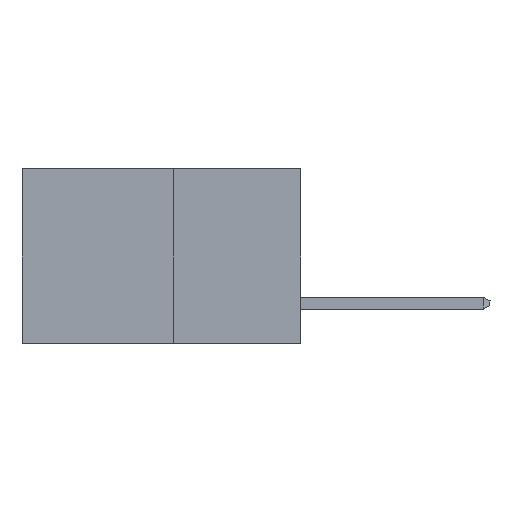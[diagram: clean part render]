
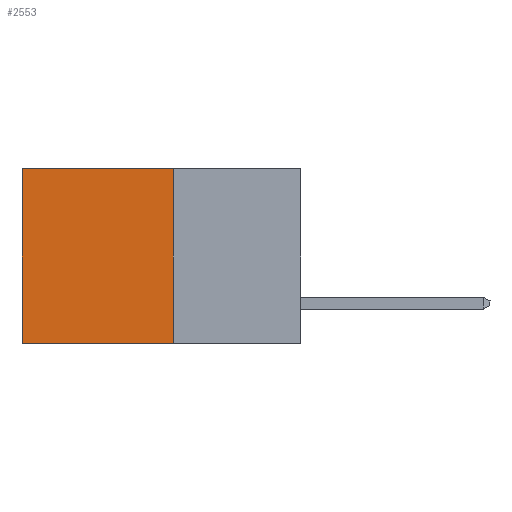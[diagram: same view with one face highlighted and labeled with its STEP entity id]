
A CAD part, left-side view. The second image highlights one B-rep face of the part: STEP entity #2553.
In plain terms, the highlighted planar face has unit normal (-1, 0, 0).
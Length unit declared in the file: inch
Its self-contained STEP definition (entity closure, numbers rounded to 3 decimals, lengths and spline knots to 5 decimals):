
#209 = LINE ( 'NONE', #13636, #10905 ) ;
#876 = EDGE_CURVE ( 'NONE', #1116, #26297, #20223, .T. ) ;
#1116 = VERTEX_POINT ( 'NONE', #6637 ) ;
#1895 = VECTOR ( 'NONE', #26187, 39.37008 ) ;
#2246 = VECTOR ( 'NONE', #16918, 39.37008 ) ;
#2553 = ADVANCED_FACE ( 'NONE', ( #9293 ), #8176, .F. ) ;
#4101 = ORIENTED_EDGE ( 'NONE', *, *, #876, .F. ) ;
#5620 = CARTESIAN_POINT ( 'NONE',  ( 0.277, 0.27, -0.37 ) ) ;
#5888 = DIRECTION ( 'NONE',  ( 0., 0., -1. ) ) ;
#6032 = CARTESIAN_POINT ( 'NONE',  ( 0.277, 0.27, 0. ) ) ;
#6637 = CARTESIAN_POINT ( 'NONE',  ( 0.277, 0.27, 0. ) ) ;
#7796 = ORIENTED_EDGE ( 'NONE', *, *, #14013, .F. ) ;
#7887 = EDGE_CURVE ( 'NONE', #14199, #18942, #19100, .T. ) ;
#8090 = EDGE_LOOP ( 'NONE', ( #9968, #7796, #4101, #16827 ) ) ;
#8176 = PLANE ( 'NONE',  #21762 ) ;
#9293 = FACE_OUTER_BOUND ( 'NONE', #8090, .T. ) ;
#9968 = ORIENTED_EDGE ( 'NONE', *, *, #7887, .T. ) ;
#10905 = VECTOR ( 'NONE', #24751, 39.37008 ) ;
#12193 = DIRECTION ( 'NONE',  ( 1., 0., 0. ) ) ;
#13636 = CARTESIAN_POINT ( 'NONE',  ( 0.277, 0.27, -0.37 ) ) ;
#13914 = LINE ( 'NONE', #6032, #1895 ) ;
#14013 = EDGE_CURVE ( 'NONE', #26297, #18942, #209, .T. ) ;
#14199 = VERTEX_POINT ( 'NONE', #14316 ) ;
#14316 = CARTESIAN_POINT ( 'NONE',  ( 0.277, 0.59, 0. ) ) ;
#14522 = VECTOR ( 'NONE', #5888, 39.37008 ) ;
#16519 = EDGE_CURVE ( 'NONE', #1116, #14199, #13914, .T. ) ;
#16663 = DIRECTION ( 'NONE',  ( 0., 0., -1. ) ) ;
#16771 = CARTESIAN_POINT ( 'NONE',  ( 0.277, 0.27, -0.37 ) ) ;
#16827 = ORIENTED_EDGE ( 'NONE', *, *, #16519, .T. ) ;
#16918 = DIRECTION ( 'NONE',  ( 0., 0., -1. ) ) ;
#18942 = VERTEX_POINT ( 'NONE', #25790 ) ;
#19100 = LINE ( 'NONE', #19384, #14522 ) ;
#19384 = CARTESIAN_POINT ( 'NONE',  ( 0.277, 0.59, -0.37 ) ) ;
#20123 = CARTESIAN_POINT ( 'NONE',  ( 0.277, 0.27, -0.37 ) ) ;
#20223 = LINE ( 'NONE', #16771, #2246 ) ;
#21762 = AXIS2_PLACEMENT_3D ( 'NONE', #5620, #12193, #16663 ) ;
#24751 = DIRECTION ( 'NONE',  ( 0., 1., 0. ) ) ;
#25790 = CARTESIAN_POINT ( 'NONE',  ( 0.277, 0.59, -0.37 ) ) ;
#26187 = DIRECTION ( 'NONE',  ( 0., 1., 0. ) ) ;
#26297 = VERTEX_POINT ( 'NONE', #20123 ) ;
